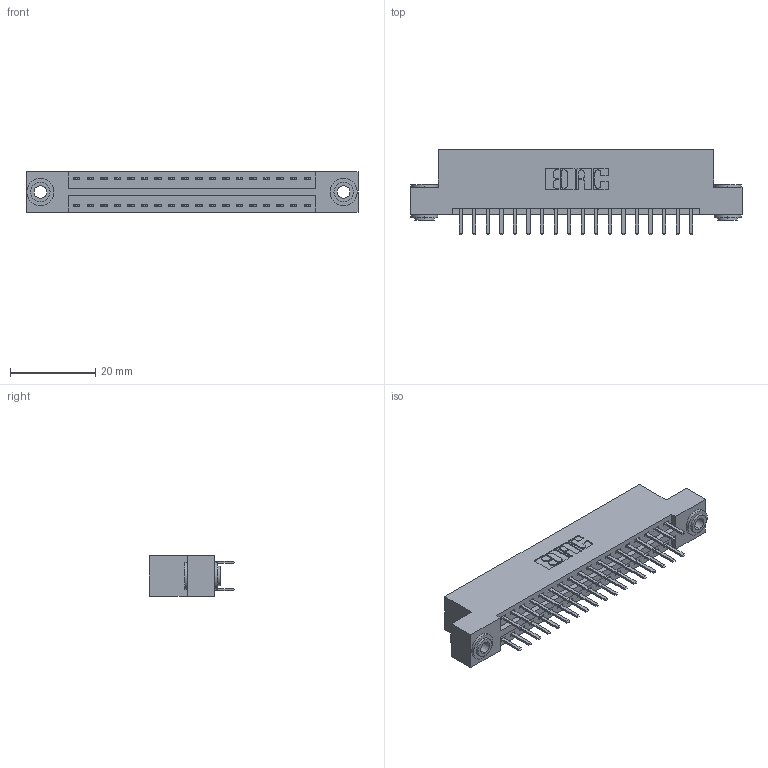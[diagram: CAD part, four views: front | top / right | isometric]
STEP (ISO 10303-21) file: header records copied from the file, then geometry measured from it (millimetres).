
FILE_DESCRIPTION (( 'STEP AP203' ), '1' );
FILE_NAME ('396-036-520-203.STEP', '2019-10-30T07:15:31', ( '' ), ( '' ), 'SwSTEP 2.0', 'SolidWorks 2016', '' );
FILE_SCHEMA (( 'CONFIG_CONTROL_DESIGN' ));
Length unit declared in the file: inch
Products named in the file (4): 345-292-001_345-293-120; 396-036-520-203; 346 Part_Flush Mounting Lugs - 0.156 Dia-TH; 345-250-002_345-250-002-102
Assembly tree (39 placements, depth 2):
  396-036-520-203
    346 Part_Flush Mounting Lugs - 0.156 Dia-TH
    345-292-001_345-293-120  x36
    345-250-002_345-250-002-102  x2
Bounding box: 77.72 x 20.02 x 9.4 mm (x, y, z)
Volume: 7396.2 mm3; surface area: 9966.5 mm2
Topology: 39 solids, 39 shells, 2176 faces, 6273 edges, 4082 vertices
Faces by surface type: plane 1418, cylinder 750, cone 8
Entity records: 15742 total; most frequent: CARTESIAN_POINT 2615, ORIENTED_EDGE 2530, DIRECTION 2375, EDGE_CURVE 1265, LINE 1033, VECTOR 1033, VERTEX_POINT 838, AXIS2_PLACEMENT_3D 671
